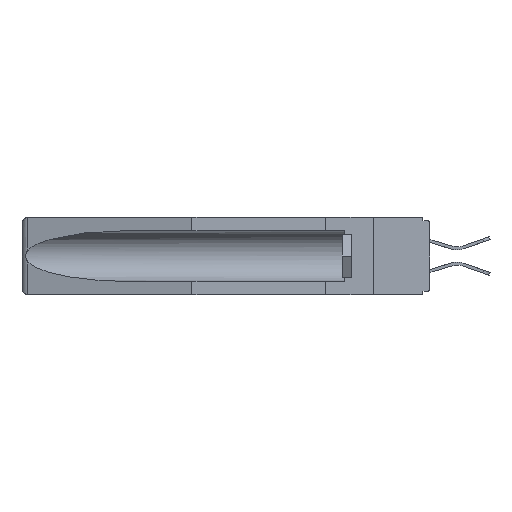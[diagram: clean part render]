
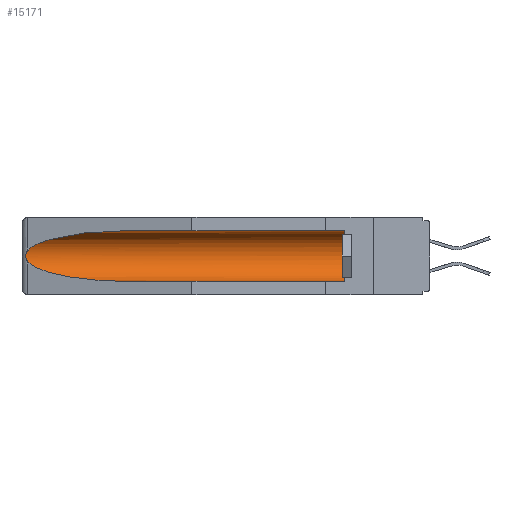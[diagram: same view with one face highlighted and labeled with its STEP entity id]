
A CAD part, left-side view. The second image highlights one B-rep face of the part: STEP entity #15171.
In plain terms, the highlighted cylindrical face has radius 2.857 mm (diameter 5.715 mm), a partial arc.
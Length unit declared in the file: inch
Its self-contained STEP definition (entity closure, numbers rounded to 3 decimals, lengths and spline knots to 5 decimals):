
#113 = ORIENTED_EDGE ( 'NONE', *, *, #15666, .T. ) ;
#234 = ORIENTED_EDGE ( 'NONE', *, *, #22068, .T. ) ;
#491 = CARTESIAN_POINT ( 'NONE',  ( 0.2675, 1.53308, -0.17534 ) ) ;
#612 = LINE ( 'NONE', #10775, #8204 ) ;
#1025 = CARTESIAN_POINT ( 'NONE',  ( 0.25451, 1.48313, -0.24835 ) ) ;
#1491 = DIRECTION ( 'NONE',  ( 0., 1., 0. ) ) ;
#1569 = DIRECTION ( 'NONE',  ( 0., 0., 1. ) ) ;
#1714 = ORIENTED_EDGE ( 'NONE', *, *, #12030, .T. ) ;
#1954 = VERTEX_POINT ( 'NONE', #9952 ) ;
#2097 = CARTESIAN_POINT ( 'NONE',  ( 0.26655, 1.53094, -0.18657 ) ) ;
#2430 = VERTEX_POINT ( 'NONE', #15366 ) ;
#2447 = CARTESIAN_POINT ( 'NONE',  ( 0.26537, 1.52718, -0.14972 ) ) ;
#2987 = B_SPLINE_CURVE_WITH_KNOTS ( 'NONE', 3,
 ( #11817, #13587, #19212, #20781, #21250, #491, #10758, #2097, #21400, #12665 ),
 .UNSPECIFIED., .F., .F.,
 ( 4, 2, 2, 2, 4 ),
 ( 0., 0.00029, 0.00058, 0.00087, 0.00117 ),
 .UNSPECIFIED. ) ;
#3374 = VECTOR ( 'NONE', #18923, 39.37008 ) ;
#3695 =( BOUNDED_CURVE ( )  B_SPLINE_CURVE ( 3, ( #7773, #9601, #11279, #2447 ),
 .UNSPECIFIED., .F., .F. ) 
 B_SPLINE_CURVE_WITH_KNOTS ( ( 4, 4 ),
 ( 4.71239, 6.08839 ),
 .UNSPECIFIED. ) 
 CURVE ( )  GEOMETRIC_REPRESENTATION_ITEM ( )  RATIONAL_B_SPLINE_CURVE ( ( 1., 0.848, 0.848, 1. ) ) 
 REPRESENTATION_ITEM ( '' )  );
#3714 = CARTESIAN_POINT ( 'NONE',  ( 0.26537, 1.52718, -0.14972 ) ) ;
#3907 = DIRECTION ( 'NONE',  ( 0., 1., 0. ) ) ;
#5101 = AXIS2_PLACEMENT_3D ( 'NONE', #14881, #13125, #16662 ) ;
#6539 = CARTESIAN_POINT ( 'NONE',  ( 0.155, 1.07973, -0.284 ) ) ;
#7731 = EDGE_CURVE ( 'NONE', #1954, #15870, #22064, .T. ) ;
#7773 = CARTESIAN_POINT ( 'NONE',  ( 0.155, 1.07973, -0.059 ) ) ;
#8204 = VECTOR ( 'NONE', #3907, 39.37008 ) ;
#8485 = CYLINDRICAL_SURFACE ( 'NONE', #9613, 0.1125 ) ;
#9601 = CARTESIAN_POINT ( 'NONE',  ( 0.21114, 1.30732, -0.059 ) ) ;
#9613 = AXIS2_PLACEMENT_3D ( 'NONE', #10156, #1491, #1569 ) ;
#9769 = ORIENTED_EDGE ( 'NONE', *, *, #20881, .T. ) ;
#9952 = CARTESIAN_POINT ( 'NONE',  ( 0.155, 0.126, -0.284 ) ) ;
#10107 =( BOUNDED_CURVE ( )  B_SPLINE_CURVE ( 3, ( #21914, #1025, #16803, #6539 ),
 .UNSPECIFIED., .F., .F. ) 
 B_SPLINE_CURVE_WITH_KNOTS ( ( 4, 4 ),
 ( 0.1948, 1.5708 ),
 .UNSPECIFIED. ) 
 CURVE ( )  GEOMETRIC_REPRESENTATION_ITEM ( )  RATIONAL_B_SPLINE_CURVE ( ( 1., 0.848, 0.848, 1. ) ) 
 REPRESENTATION_ITEM ( '' )  );
#10112 = ORIENTED_EDGE ( 'NONE', *, *, #7731, .T. ) ;
#10156 = CARTESIAN_POINT ( 'NONE',  ( 0.155, -0.30754, -0.1715 ) ) ;
#10758 = CARTESIAN_POINT ( 'NONE',  ( 0.2673, 1.53269, -0.17917 ) ) ;
#10775 = CARTESIAN_POINT ( 'NONE',  ( 0.155, -0.30754, -0.059 ) ) ;
#11279 = CARTESIAN_POINT ( 'NONE',  ( 0.25451, 1.48313, -0.09465 ) ) ;
#11796 = CARTESIAN_POINT ( 'NONE',  ( 0.155, 1.07973, -0.059 ) ) ;
#11817 = CARTESIAN_POINT ( 'NONE',  ( 0.26537, 1.52718, -0.14972 ) ) ;
#12030 = EDGE_CURVE ( 'NONE', #16134, #12449, #3695, .T. ) ;
#12449 = VERTEX_POINT ( 'NONE', #3714 ) ;
#12665 = CARTESIAN_POINT ( 'NONE',  ( 0.26537, 1.52718, -0.19328 ) ) ;
#12988 = CARTESIAN_POINT ( 'NONE',  ( 0.155, 1.07973, -0.284 ) ) ;
#13125 = DIRECTION ( 'NONE',  ( 0., -1., 0. ) ) ;
#13258 = VERTEX_POINT ( 'NONE', #12988 ) ;
#13587 = CARTESIAN_POINT ( 'NONE',  ( 0.26597, 1.52961, -0.15275 ) ) ;
#13889 = EDGE_CURVE ( 'NONE', #1954, #13258, #16240, .T. ) ;
#14673 = EDGE_LOOP ( 'NONE', ( #1714, #9769, #234, #21717, #10112, #113 ) ) ;
#14881 = CARTESIAN_POINT ( 'NONE',  ( 0.155, 0.126, -0.1715 ) ) ;
#15171 = ADVANCED_FACE ( 'NONE', ( #18919 ), #8485, .F. ) ;
#15366 = CARTESIAN_POINT ( 'NONE',  ( 0.26537, 1.52718, -0.19328 ) ) ;
#15666 = EDGE_CURVE ( 'NONE', #15870, #16134, #612, .T. ) ;
#15870 = VERTEX_POINT ( 'NONE', #20425 ) ;
#16134 = VERTEX_POINT ( 'NONE', #11796 ) ;
#16240 = LINE ( 'NONE', #18849, #3374 ) ;
#16662 = DIRECTION ( 'NONE',  ( 0., 0., 1. ) ) ;
#16803 = CARTESIAN_POINT ( 'NONE',  ( 0.21114, 1.30732, -0.284 ) ) ;
#18849 = CARTESIAN_POINT ( 'NONE',  ( 0.155, -0.30754, -0.284 ) ) ;
#18919 = FACE_OUTER_BOUND ( 'NONE', #14673, .T. ) ;
#18923 = DIRECTION ( 'NONE',  ( 0., 1., 0. ) ) ;
#19212 = CARTESIAN_POINT ( 'NONE',  ( 0.26654, 1.53092, -0.15636 ) ) ;
#20425 = CARTESIAN_POINT ( 'NONE',  ( 0.155, 0.126, -0.059 ) ) ;
#20781 = CARTESIAN_POINT ( 'NONE',  ( 0.2673, 1.5327, -0.16383 ) ) ;
#20881 = EDGE_CURVE ( 'NONE', #12449, #2430, #2987, .T. ) ;
#21250 = CARTESIAN_POINT ( 'NONE',  ( 0.2675, 1.53308, -0.16763 ) ) ;
#21400 = CARTESIAN_POINT ( 'NONE',  ( 0.26597, 1.5296, -0.19026 ) ) ;
#21717 = ORIENTED_EDGE ( 'NONE', *, *, #13889, .F. ) ;
#21914 = CARTESIAN_POINT ( 'NONE',  ( 0.26537, 1.52718, -0.19328 ) ) ;
#22064 = CIRCLE ( 'NONE', #5101, 0.1125 ) ;
#22068 = EDGE_CURVE ( 'NONE', #2430, #13258, #10107, .T. ) ;
